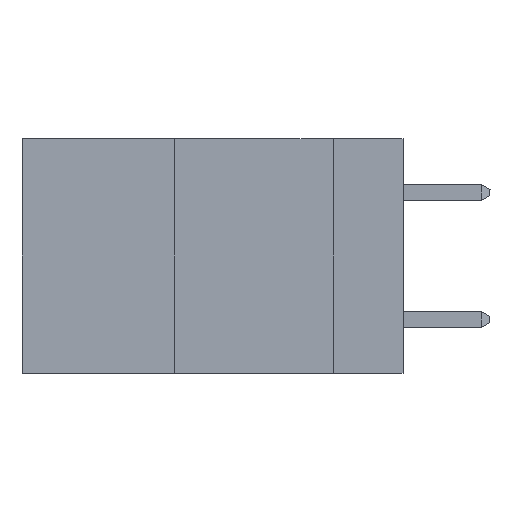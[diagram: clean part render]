
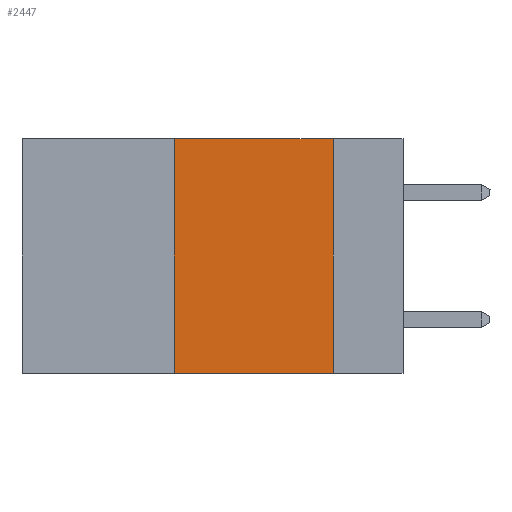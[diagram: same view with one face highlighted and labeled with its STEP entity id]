
A CAD part, left-side view. The second image highlights one B-rep face of the part: STEP entity #2447.
In plain terms, the highlighted planar face has unit normal (-1, 0, 0).
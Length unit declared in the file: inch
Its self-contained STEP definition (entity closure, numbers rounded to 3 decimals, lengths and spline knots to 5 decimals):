
#1033 = CARTESIAN_POINT ( 'NONE',  ( 0., 0.36, -0.37 ) ) ;
#1621 = CARTESIAN_POINT ( 'NONE',  ( 0., 0.11, 0. ) ) ;
#1906 = CARTESIAN_POINT ( 'NONE',  ( 0., 0.36, 0. ) ) ;
#2447 = ADVANCED_FACE ( 'NONE', ( #5758 ), #7157, .F. ) ;
#2963 = CARTESIAN_POINT ( 'NONE',  ( 0., 0.6, 0. ) ) ;
#3115 = DIRECTION ( 'NONE',  ( 1., 0., 0. ) ) ;
#4491 = LINE ( 'NONE', #1906, #6951 ) ;
#4876 = VECTOR ( 'NONE', #14647, 39.37008 ) ;
#5495 = DIRECTION ( 'NONE',  ( 0., 0., -1. ) ) ;
#5758 = FACE_OUTER_BOUND ( 'NONE', #20329, .T. ) ;
#6305 = DIRECTION ( 'NONE',  ( 0., 0., 1. ) ) ;
#6951 = VECTOR ( 'NONE', #6305, 39.37008 ) ;
#7157 = PLANE ( 'NONE',  #22451 ) ;
#8297 = DIRECTION ( 'NONE',  ( 0., -1., 0. ) ) ;
#8511 = CARTESIAN_POINT ( 'NONE',  ( 0., 0.11, 0. ) ) ;
#9908 = ORIENTED_EDGE ( 'NONE', *, *, #13326, .F. ) ;
#10008 = DIRECTION ( 'NONE',  ( 0., -1., 0. ) ) ;
#10080 = EDGE_CURVE ( 'NONE', #12918, #28417, #14482, .T. ) ;
#10265 = EDGE_CURVE ( 'NONE', #22898, #26326, #4491, .T. ) ;
#10609 = CARTESIAN_POINT ( 'NONE',  ( 0., 0.6, -0.37 ) ) ;
#12316 = ORIENTED_EDGE ( 'NONE', *, *, #22429, .T. ) ;
#12537 = ORIENTED_EDGE ( 'NONE', *, *, #10265, .F. ) ;
#12918 = VERTEX_POINT ( 'NONE', #8511 ) ;
#13301 = ORIENTED_EDGE ( 'NONE', *, *, #10080, .F. ) ;
#13326 = EDGE_CURVE ( 'NONE', #26326, #12918, #15195, .T. ) ;
#13777 = VECTOR ( 'NONE', #10008, 39.37008 ) ;
#14482 = LINE ( 'NONE', #1621, #4876 ) ;
#14617 = CARTESIAN_POINT ( 'NONE',  ( 0., 0.6, 0. ) ) ;
#14647 = DIRECTION ( 'NONE',  ( 0., 0., -1. ) ) ;
#15195 = LINE ( 'NONE', #2963, #13777 ) ;
#15878 = CARTESIAN_POINT ( 'NONE',  ( 0., 0.36, 0. ) ) ;
#20329 = EDGE_LOOP ( 'NONE', ( #13301, #9908, #12537, #12316 ) ) ;
#22278 = VECTOR ( 'NONE', #8297, 39.37008 ) ;
#22429 = EDGE_CURVE ( 'NONE', #22898, #28417, #28975, .T. ) ;
#22451 = AXIS2_PLACEMENT_3D ( 'NONE', #14617, #3115, #5495 ) ;
#22898 = VERTEX_POINT ( 'NONE', #1033 ) ;
#23419 = CARTESIAN_POINT ( 'NONE',  ( 0., 0.11, -0.37 ) ) ;
#26326 = VERTEX_POINT ( 'NONE', #15878 ) ;
#28417 = VERTEX_POINT ( 'NONE', #23419 ) ;
#28975 = LINE ( 'NONE', #10609, #22278 ) ;
